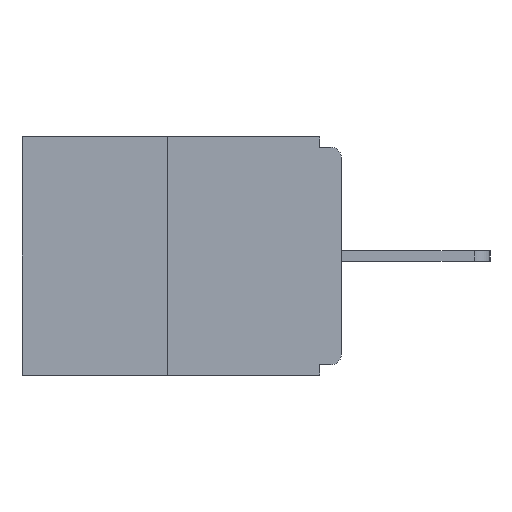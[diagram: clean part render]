
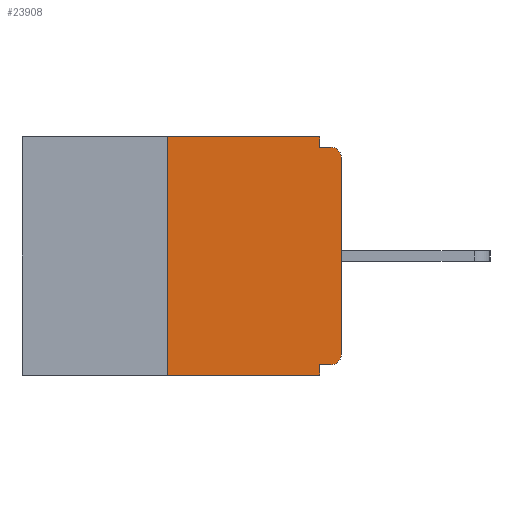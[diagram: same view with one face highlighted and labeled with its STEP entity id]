
A CAD part, left-side view. The second image highlights one B-rep face of the part: STEP entity #23908.
In plain terms, the highlighted planar face has unit normal (-1, 0, 0).
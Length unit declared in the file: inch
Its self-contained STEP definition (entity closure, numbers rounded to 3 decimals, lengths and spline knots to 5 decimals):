
#89 = VERTEX_POINT ( 'NONE', #5135 ) ;
#173 = CARTESIAN_POINT ( 'NONE',  ( 0., 0., -0.03 ) ) ;
#605 = CARTESIAN_POINT ( 'NONE',  ( 0., 0., 0. ) ) ;
#745 = EDGE_CURVE ( 'NONE', #89, #24960, #15213, .T. ) ;
#1042 = DIRECTION ( 'NONE',  ( 0., 0., -1. ) ) ;
#1485 = EDGE_CURVE ( 'NONE', #12920, #19254, #23090, .T. ) ;
#2353 = LINE ( 'NONE', #6061, #26559 ) ;
#2436 = DIRECTION ( 'NONE',  ( 0., 0., 1. ) ) ;
#2596 = LINE ( 'NONE', #14629, #27487 ) ;
#2654 = CARTESIAN_POINT ( 'NONE',  ( 0., 0.015, -0.03 ) ) ;
#2955 = CARTESIAN_POINT ( 'NONE',  ( 0., 0.25, -0.343 ) ) ;
#2993 = DIRECTION ( 'NONE',  ( 1., 0., 0. ) ) ;
#3017 = VECTOR ( 'NONE', #11315, 39.37008 ) ;
#3661 = CARTESIAN_POINT ( 'NONE',  ( 0., 0.015, -0.313 ) ) ;
#4556 = VERTEX_POINT ( 'NONE', #14354 ) ;
#4889 = DIRECTION ( 'NONE',  ( 0., 0., -1. ) ) ;
#5135 = CARTESIAN_POINT ( 'NONE',  ( 0., 0.031, -0.328 ) ) ;
#5991 = EDGE_CURVE ( 'NONE', #13022, #26938, #12117, .T. ) ;
#6061 = CARTESIAN_POINT ( 'NONE',  ( 0., 0.031, 0. ) ) ;
#7104 = DIRECTION ( 'NONE',  ( 0., 0., -1. ) ) ;
#7537 = VECTOR ( 'NONE', #2436, 39.37008 ) ;
#7644 = CARTESIAN_POINT ( 'NONE',  ( 0., 0.46, -0.343 ) ) ;
#8050 = DIRECTION ( 'NONE',  ( -1., 0., 0. ) ) ;
#8283 = CARTESIAN_POINT ( 'NONE',  ( 0., 0.015, -0.328 ) ) ;
#8460 = EDGE_CURVE ( 'NONE', #12920, #89, #2596, .T. ) ;
#8550 = LINE ( 'NONE', #11163, #7537 ) ;
#8644 = ORIENTED_EDGE ( 'NONE', *, *, #1485, .T. ) ;
#8976 = ORIENTED_EDGE ( 'NONE', *, *, #25877, .F. ) ;
#9328 = PLANE ( 'NONE',  #26351 ) ;
#9994 = AXIS2_PLACEMENT_3D ( 'NONE', #3661, #8050, #27233 ) ;
#10027 = LINE ( 'NONE', #13082, #20621 ) ;
#10232 = ORIENTED_EDGE ( 'NONE', *, *, #745, .F. ) ;
#10535 = ORIENTED_EDGE ( 'NONE', *, *, #17394, .T. ) ;
#11163 = CARTESIAN_POINT ( 'NONE',  ( 0., 0.25, 0. ) ) ;
#11315 = DIRECTION ( 'NONE',  ( 0., 0., 1. ) ) ;
#11436 = EDGE_CURVE ( 'NONE', #14189, #12101, #8550, .T. ) ;
#12011 = ORIENTED_EDGE ( 'NONE', *, *, #14520, .F. ) ;
#12101 = VERTEX_POINT ( 'NONE', #21198 ) ;
#12117 = CIRCLE ( 'NONE', #16527, 0.015 ) ;
#12873 = DIRECTION ( 'NONE',  ( 0., 0., -1. ) ) ;
#12920 = VERTEX_POINT ( 'NONE', #8283 ) ;
#13022 = VERTEX_POINT ( 'NONE', #173 ) ;
#13082 = CARTESIAN_POINT ( 'NONE',  ( 0., 0.46, 0. ) ) ;
#13375 = LINE ( 'NONE', #605, #3017 ) ;
#13780 = EDGE_CURVE ( 'NONE', #19254, #13022, #13375, .T. ) ;
#13941 = VECTOR ( 'NONE', #19571, 39.37008 ) ;
#13993 = DIRECTION ( 'NONE',  ( 0., -1., 0. ) ) ;
#14189 = VERTEX_POINT ( 'NONE', #2955 ) ;
#14303 = LINE ( 'NONE', #17442, #13941 ) ;
#14354 = CARTESIAN_POINT ( 'NONE',  ( 0., 0.031, -0.015 ) ) ;
#14520 = EDGE_CURVE ( 'NONE', #4556, #26938, #14303, .T. ) ;
#14629 = CARTESIAN_POINT ( 'NONE',  ( 0., 0., -0.328 ) ) ;
#15213 = LINE ( 'NONE', #21624, #23110 ) ;
#15328 = DIRECTION ( 'NONE',  ( -1., 0., 0. ) ) ;
#15493 = CARTESIAN_POINT ( 'NONE',  ( 0., 0., -0.313 ) ) ;
#16297 = CARTESIAN_POINT ( 'NONE',  ( 0., 0.031, -0.343 ) ) ;
#16527 = AXIS2_PLACEMENT_3D ( 'NONE', #2654, #15328, #7104 ) ;
#16598 = CARTESIAN_POINT ( 'NONE',  ( 0., 0.031, 0. ) ) ;
#17394 = EDGE_CURVE ( 'NONE', #14189, #24960, #23129, .T. ) ;
#17442 = CARTESIAN_POINT ( 'NONE',  ( 0., 0., -0.015 ) ) ;
#18506 = VECTOR ( 'NONE', #13993, 39.37008 ) ;
#18616 = ORIENTED_EDGE ( 'NONE', *, *, #5991, .T. ) ;
#19254 = VERTEX_POINT ( 'NONE', #15493 ) ;
#19297 = EDGE_LOOP ( 'NONE', ( #22963, #24473, #10535, #10232, #22600, #8644, #20301, #18616, #12011, #8976 ) ) ;
#19571 = DIRECTION ( 'NONE',  ( 0., -1., 0. ) ) ;
#19617 = DIRECTION ( 'NONE',  ( 0., -1., 0. ) ) ;
#20301 = ORIENTED_EDGE ( 'NONE', *, *, #13780, .T. ) ;
#20374 = EDGE_CURVE ( 'NONE', #12101, #25855, #10027, .T. ) ;
#20621 = VECTOR ( 'NONE', #19617, 39.37008 ) ;
#21198 = CARTESIAN_POINT ( 'NONE',  ( 0., 0.25, 0. ) ) ;
#21342 = DIRECTION ( 'NONE',  ( 0., 1., 0. ) ) ;
#21474 = CARTESIAN_POINT ( 'NONE',  ( 0., 0.015, -0.015 ) ) ;
#21624 = CARTESIAN_POINT ( 'NONE',  ( 0., 0.031, -0.343 ) ) ;
#22276 = CARTESIAN_POINT ( 'NONE',  ( 0., 0.46, 0. ) ) ;
#22600 = ORIENTED_EDGE ( 'NONE', *, *, #8460, .F. ) ;
#22963 = ORIENTED_EDGE ( 'NONE', *, *, #20374, .F. ) ;
#23090 = CIRCLE ( 'NONE', #9994, 0.015 ) ;
#23110 = VECTOR ( 'NONE', #4889, 39.37008 ) ;
#23129 = LINE ( 'NONE', #7644, #18506 ) ;
#23733 = FACE_OUTER_BOUND ( 'NONE', #19297, .T. ) ;
#23908 = ADVANCED_FACE ( 'NONE', ( #23733 ), #9328, .F. ) ;
#24473 = ORIENTED_EDGE ( 'NONE', *, *, #11436, .F. ) ;
#24960 = VERTEX_POINT ( 'NONE', #16297 ) ;
#25855 = VERTEX_POINT ( 'NONE', #16598 ) ;
#25877 = EDGE_CURVE ( 'NONE', #25855, #4556, #2353, .T. ) ;
#26351 = AXIS2_PLACEMENT_3D ( 'NONE', #22276, #2993, #1042 ) ;
#26559 = VECTOR ( 'NONE', #12873, 39.37008 ) ;
#26938 = VERTEX_POINT ( 'NONE', #21474 ) ;
#27233 = DIRECTION ( 'NONE',  ( 0., 0., -1. ) ) ;
#27487 = VECTOR ( 'NONE', #21342, 39.37008 ) ;
